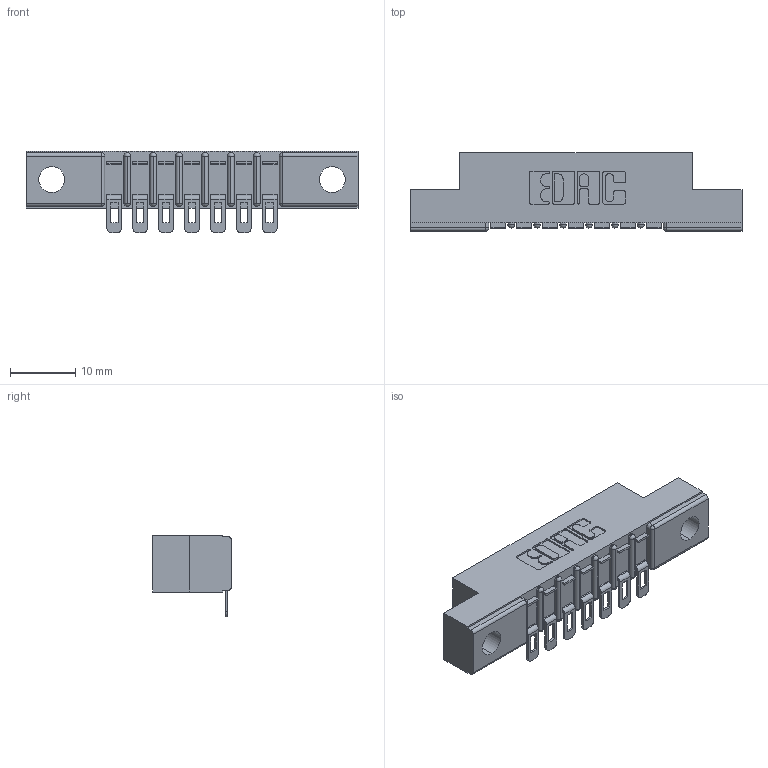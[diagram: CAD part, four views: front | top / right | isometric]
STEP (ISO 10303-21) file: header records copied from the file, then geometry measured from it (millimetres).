
FILE_DESCRIPTION (( 'STEP AP203' ), '1' );
FILE_NAME ('307-007-454-104.STEP', '2020-09-25T02:39:01', ( '' ), ( '' ), 'SwSTEP 2.0', 'SolidWorks 2020', '' );
FILE_SCHEMA (( 'CONFIG_CONTROL_DESIGN' ));
Length unit declared in the file: inch
Products named in the file (3): 307 Part_.156 Dia Mounting Holes; 307-290-002_554; 307-007-454-104
Assembly tree (8 placements, depth 2):
  307-007-454-104
    307 Part_.156 Dia Mounting Holes
    307-290-002_554  x7
Bounding box: 50.75 x 12.01 x 12.52 mm (x, y, z)
Volume: 3239.1 mm3; surface area: 4976.9 mm2
Topology: 8 solids, 8 shells, 707 faces, 2130 edges, 1396 vertices
Faces by surface type: plane 406, cylinder 285, sphere 16
Entity records: 11699 total; most frequent: CARTESIAN_POINT 1972, ORIENTED_EDGE 1960, DIRECTION 1930, EDGE_CURVE 980, VECTOR 734, LINE 734, VERTEX_POINT 640, AXIS2_PLACEMENT_3D 598
